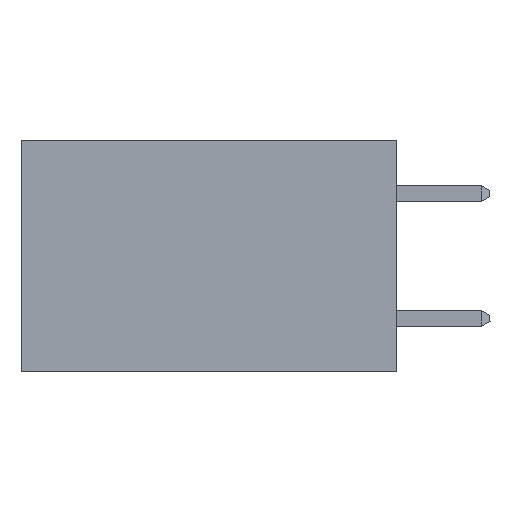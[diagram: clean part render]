
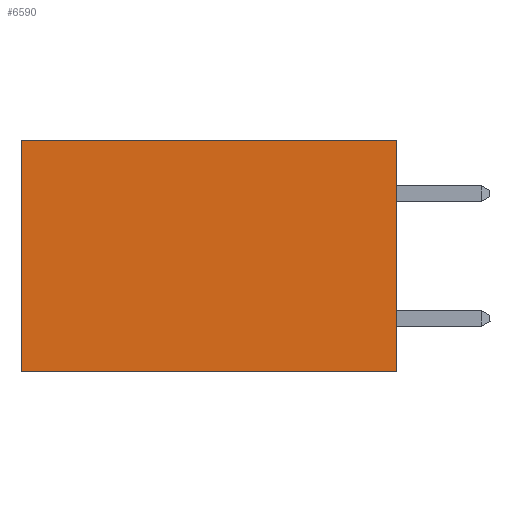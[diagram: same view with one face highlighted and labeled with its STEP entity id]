
A CAD part, left-side view. The second image highlights one B-rep face of the part: STEP entity #6590.
In plain terms, the highlighted planar face has unit normal (-1, 0, 0).
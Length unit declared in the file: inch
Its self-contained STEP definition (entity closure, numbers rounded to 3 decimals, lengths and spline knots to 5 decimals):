
#906 = EDGE_CURVE ( 'NONE', #2574, #4953, #1923, .T. ) ;
#1120 = VECTOR ( 'NONE', #2232, 39.37008 ) ;
#1743 = VERTEX_POINT ( 'NONE', #4696 ) ;
#1923 = LINE ( 'NONE', #8082, #3789 ) ;
#1963 = LINE ( 'NONE', #2327, #1120 ) ;
#2232 = DIRECTION ( 'NONE',  ( 0., 1., 0. ) ) ;
#2307 = CARTESIAN_POINT ( 'NONE',  ( 0.2615, 0., -0.37 ) ) ;
#2327 = CARTESIAN_POINT ( 'NONE',  ( 0.2615, 0., 0. ) ) ;
#2574 = VERTEX_POINT ( 'NONE', #4756 ) ;
#2589 = DIRECTION ( 'NONE',  ( 0., 0., -1. ) ) ;
#3220 = CARTESIAN_POINT ( 'NONE',  ( 0.2615, 0.6, -0.37 ) ) ;
#3318 = AXIS2_PLACEMENT_3D ( 'NONE', #4188, #8621, #2589 ) ;
#3476 = DIRECTION ( 'NONE',  ( 0., 0., -1. ) ) ;
#3704 = VERTEX_POINT ( 'NONE', #2307 ) ;
#3767 = EDGE_CURVE ( 'NONE', #3704, #4953, #8929, .T. ) ;
#3789 = VECTOR ( 'NONE', #3476, 39.37008 ) ;
#3802 = EDGE_CURVE ( 'NONE', #1743, #3704, #4818, .T. ) ;
#3930 = ORIENTED_EDGE ( 'NONE', *, *, #3767, .F. ) ;
#3937 = DIRECTION ( 'NONE',  ( 0., 1., 0. ) ) ;
#4188 = CARTESIAN_POINT ( 'NONE',  ( 0.2615, 0., -0.37 ) ) ;
#4566 = VECTOR ( 'NONE', #6929, 39.37008 ) ;
#4696 = CARTESIAN_POINT ( 'NONE',  ( 0.2615, 0., 0. ) ) ;
#4756 = CARTESIAN_POINT ( 'NONE',  ( 0.2615, 0.6, 0. ) ) ;
#4818 = LINE ( 'NONE', #6267, #4566 ) ;
#4953 = VERTEX_POINT ( 'NONE', #3220 ) ;
#6015 = EDGE_LOOP ( 'NONE', ( #9555, #3930, #6201, #7959 ) ) ;
#6186 = EDGE_CURVE ( 'NONE', #1743, #2574, #1963, .T. ) ;
#6201 = ORIENTED_EDGE ( 'NONE', *, *, #3802, .F. ) ;
#6267 = CARTESIAN_POINT ( 'NONE',  ( 0.2615, 0., -0.37 ) ) ;
#6590 = ADVANCED_FACE ( 'NONE', ( #7616 ), #7888, .F. ) ;
#6929 = DIRECTION ( 'NONE',  ( 0., 0., -1. ) ) ;
#7616 = FACE_OUTER_BOUND ( 'NONE', #6015, .T. ) ;
#7888 = PLANE ( 'NONE',  #3318 ) ;
#7959 = ORIENTED_EDGE ( 'NONE', *, *, #6186, .T. ) ;
#8082 = CARTESIAN_POINT ( 'NONE',  ( 0.2615, 0.6, -0.37 ) ) ;
#8233 = VECTOR ( 'NONE', #3937, 39.37008 ) ;
#8491 = CARTESIAN_POINT ( 'NONE',  ( 0.2615, 0., -0.37 ) ) ;
#8621 = DIRECTION ( 'NONE',  ( 1., 0., 0. ) ) ;
#8929 = LINE ( 'NONE', #8491, #8233 ) ;
#9555 = ORIENTED_EDGE ( 'NONE', *, *, #906, .T. ) ;
